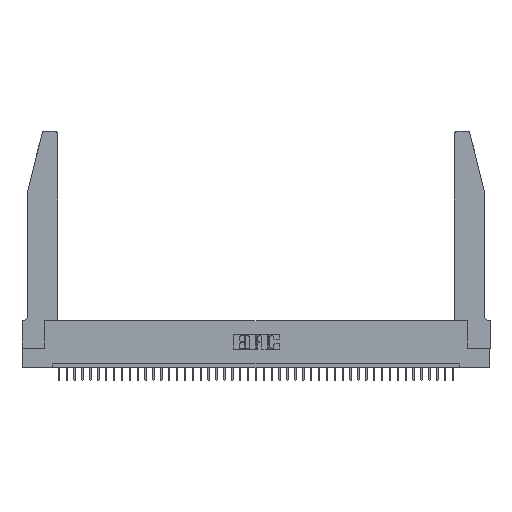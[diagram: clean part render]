
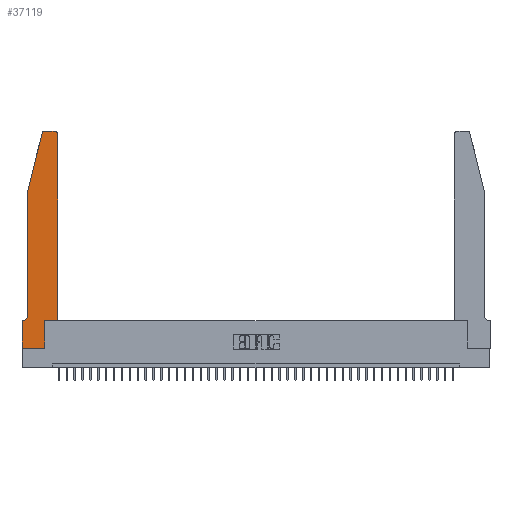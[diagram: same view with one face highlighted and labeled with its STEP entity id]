
A CAD part, top view. The second image highlights one B-rep face of the part: STEP entity #37119.
In plain terms, the highlighted planar face has unit normal (0, 0, 1).
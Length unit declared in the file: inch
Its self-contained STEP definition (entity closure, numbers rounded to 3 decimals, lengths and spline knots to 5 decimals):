
#324 = ORIENTED_EDGE ( 'NONE', *, *, #33193, .T. ) ;
#956 = CARTESIAN_POINT ( 'NONE',  ( 0.2865, 0.35, 0.37 ) ) ;
#963 = EDGE_CURVE ( 'NONE', #12908, #16970, #10690, .T. ) ;
#1066 = CARTESIAN_POINT ( 'NONE',  ( 0., 0., 0.37 ) ) ;
#1151 = CARTESIAN_POINT ( 'NONE',  ( 0., 0., 0.37 ) ) ;
#1848 = VECTOR ( 'NONE', #27713, 39.37008 ) ;
#1922 = DIRECTION ( 'NONE',  ( -1., 0., 0. ) ) ;
#2053 = VERTEX_POINT ( 'NONE', #23676 ) ;
#2090 = EDGE_CURVE ( 'NONE', #25463, #10935, #2439, .T. ) ;
#2155 = CARTESIAN_POINT ( 'NONE',  ( 0.2865, 0.35, 0.37 ) ) ;
#2161 = CARTESIAN_POINT ( 'NONE',  ( 0.0755, 2., 0.37 ) ) ;
#2421 = VERTEX_POINT ( 'NONE', #1151 ) ;
#2439 = CIRCLE ( 'NONE', #33643, 0.07 ) ;
#2647 = EDGE_CURVE ( 'NONE', #2421, #18058, #10616, .T. ) ;
#2859 = DIRECTION ( 'NONE',  ( 0., 0., 1. ) ) ;
#2985 = ORIENTED_EDGE ( 'NONE', *, *, #25477, .T. ) ;
#3070 = EDGE_CURVE ( 'NONE', #10935, #2053, #19215, .T. ) ;
#5065 = ORIENTED_EDGE ( 'NONE', *, *, #2647, .T. ) ;
#5070 = ORIENTED_EDGE ( 'NONE', *, *, #39161, .T. ) ;
#5489 = VECTOR ( 'NONE', #8986, 39.37008 ) ;
#5633 = VECTOR ( 'NONE', #26373, 39.37008 ) ;
#5861 = CARTESIAN_POINT ( 'NONE',  ( 0., 0., 0.37 ) ) ;
#6131 = VECTOR ( 'NONE', #7874, 39.37008 ) ;
#6667 = DIRECTION ( 'NONE',  ( 0., 0., 1. ) ) ;
#7221 = EDGE_LOOP ( 'NONE', ( #12255, #30014, #24522, #31162, #35668, #37573, #324, #5065, #5070, #12516, #27446, #2985 ) ) ;
#7874 = DIRECTION ( 'NONE',  ( 0., 1., 0. ) ) ;
#7950 = LINE ( 'NONE', #1066, #26227 ) ;
#8197 = CARTESIAN_POINT ( 'NONE',  ( 0.2865, 0., 0.37 ) ) ;
#8962 = VERTEX_POINT ( 'NONE', #33099 ) ;
#8986 = DIRECTION ( 'NONE',  ( -1., 0., 0. ) ) ;
#10113 = DIRECTION ( 'NONE',  ( 1., 0., 0. ) ) ;
#10242 = DIRECTION ( 'NONE',  ( 1., 0., 0. ) ) ;
#10523 = DIRECTION ( 'NONE',  ( 0., 0., 1. ) ) ;
#10616 = LINE ( 'NONE', #5861, #22814 ) ;
#10690 = LINE ( 'NONE', #33663, #6131 ) ;
#10935 = VERTEX_POINT ( 'NONE', #17726 ) ;
#11370 = CIRCLE ( 'NONE', #39183, 0.03 ) ;
#11614 = VERTEX_POINT ( 'NONE', #14839 ) ;
#12255 = ORIENTED_EDGE ( 'NONE', *, *, #16930, .T. ) ;
#12516 = ORIENTED_EDGE ( 'NONE', *, *, #23753, .T. ) ;
#12787 = DIRECTION ( 'NONE',  ( 1., 0., 0. ) ) ;
#12908 = VERTEX_POINT ( 'NONE', #32013 ) ;
#14839 = CARTESIAN_POINT ( 'NONE',  ( 0.25487, 2.72718, 0.37 ) ) ;
#14938 = CARTESIAN_POINT ( 'NONE',  ( 0.2605, 2.75, 0.37 ) ) ;
#15111 = CARTESIAN_POINT ( 'NONE',  ( 0.284, 2.75, 0.37 ) ) ;
#15152 = VERTEX_POINT ( 'NONE', #15111 ) ;
#15331 = DIRECTION ( 'NONE',  ( 0., -1., 0. ) ) ;
#15503 = CARTESIAN_POINT ( 'NONE',  ( 0.4505, 2.72, 0.37 ) ) ;
#16038 = CARTESIAN_POINT ( 'NONE',  ( 0.284, 2.72, 0.37 ) ) ;
#16930 = EDGE_CURVE ( 'NONE', #8962, #15152, #28844, .T. ) ;
#16970 = VERTEX_POINT ( 'NONE', #15503 ) ;
#17034 = PLANE ( 'NONE',  #22328 ) ;
#17726 = CARTESIAN_POINT ( 'NONE',  ( 0.0055, 0.35, 0.37 ) ) ;
#17908 = DIRECTION ( 'NONE',  ( 1., 0., 0. ) ) ;
#18058 = VERTEX_POINT ( 'NONE', #8197 ) ;
#19215 = LINE ( 'NONE', #30645, #26817 ) ;
#21968 = VECTOR ( 'NONE', #26940, 39.37008 ) ;
#22328 = AXIS2_PLACEMENT_3D ( 'NONE', #39568, #10523, #10242 ) ;
#22492 = CARTESIAN_POINT ( 'NONE',  ( 0.0755, 0.42, 0.37 ) ) ;
#22814 = VECTOR ( 'NONE', #17908, 39.37008 ) ;
#23544 = CARTESIAN_POINT ( 'NONE',  ( 0.0755, 2., 0.37 ) ) ;
#23676 = CARTESIAN_POINT ( 'NONE',  ( 0., 0.35, 0.37 ) ) ;
#23753 = EDGE_CURVE ( 'NONE', #27836, #12908, #27764, .T. ) ;
#23909 = LINE ( 'NONE', #23544, #5633 ) ;
#24251 = EDGE_CURVE ( 'NONE', #38512, #25463, #33740, .T. ) ;
#24522 = ORIENTED_EDGE ( 'NONE', *, *, #26906, .T. ) ;
#25158 = VECTOR ( 'NONE', #15331, 39.37008 ) ;
#25463 = VERTEX_POINT ( 'NONE', #22492 ) ;
#25477 = EDGE_CURVE ( 'NONE', #16970, #8962, #11370, .T. ) ;
#26227 = VECTOR ( 'NONE', #40353, 39.37008 ) ;
#26373 = DIRECTION ( 'NONE',  ( -0.239, -0.971, 0. ) ) ;
#26480 = CIRCLE ( 'NONE', #27012, 0.03 ) ;
#26491 = LINE ( 'NONE', #956, #21968 ) ;
#26817 = VECTOR ( 'NONE', #33894, 39.37008 ) ;
#26906 = EDGE_CURVE ( 'NONE', #11614, #38512, #23909, .T. ) ;
#26940 = DIRECTION ( 'NONE',  ( 0., 1., 0. ) ) ;
#27012 = AXIS2_PLACEMENT_3D ( 'NONE', #16038, #6667, #12787 ) ;
#27446 = ORIENTED_EDGE ( 'NONE', *, *, #963, .T. ) ;
#27713 = DIRECTION ( 'NONE',  ( 1., 0., 0. ) ) ;
#27727 = FACE_OUTER_BOUND ( 'NONE', #7221, .T. ) ;
#27764 = LINE ( 'NONE', #33781, #1848 ) ;
#27836 = VERTEX_POINT ( 'NONE', #2155 ) ;
#28844 = LINE ( 'NONE', #14938, #5489 ) ;
#30014 = ORIENTED_EDGE ( 'NONE', *, *, #41969, .T. ) ;
#30645 = CARTESIAN_POINT ( 'NONE',  ( 0.0755, 0.35, 0.37 ) ) ;
#31162 = ORIENTED_EDGE ( 'NONE', *, *, #24251, .T. ) ;
#31560 = CARTESIAN_POINT ( 'NONE',  ( 0.0055, 0.42, 0.37 ) ) ;
#32013 = CARTESIAN_POINT ( 'NONE',  ( 0.4505, 0.35, 0.37 ) ) ;
#33099 = CARTESIAN_POINT ( 'NONE',  ( 0.4205, 2.75, 0.37 ) ) ;
#33193 = EDGE_CURVE ( 'NONE', #2053, #2421, #7950, .T. ) ;
#33643 = AXIS2_PLACEMENT_3D ( 'NONE', #31560, #34250, #1922 ) ;
#33663 = CARTESIAN_POINT ( 'NONE',  ( 0.4505, 0.35, 0.37 ) ) ;
#33740 = LINE ( 'NONE', #37880, #25158 ) ;
#33781 = CARTESIAN_POINT ( 'NONE',  ( 0.4505, 0.35, 0.37 ) ) ;
#33894 = DIRECTION ( 'NONE',  ( -1., 0., 0. ) ) ;
#34250 = DIRECTION ( 'NONE',  ( 0., 0., -1. ) ) ;
#35668 = ORIENTED_EDGE ( 'NONE', *, *, #2090, .T. ) ;
#37119 = ADVANCED_FACE ( 'NONE', ( #27727 ), #17034, .T. ) ;
#37573 = ORIENTED_EDGE ( 'NONE', *, *, #3070, .T. ) ;
#37880 = CARTESIAN_POINT ( 'NONE',  ( 0.0755, 2., 0.37 ) ) ;
#38512 = VERTEX_POINT ( 'NONE', #2161 ) ;
#39161 = EDGE_CURVE ( 'NONE', #18058, #27836, #26491, .T. ) ;
#39183 = AXIS2_PLACEMENT_3D ( 'NONE', #41718, #2859, #10113 ) ;
#39568 = CARTESIAN_POINT ( 'NONE',  ( 0., 0.35, 0.37 ) ) ;
#40353 = DIRECTION ( 'NONE',  ( 0., -1., 0. ) ) ;
#41718 = CARTESIAN_POINT ( 'NONE',  ( 0.4205, 2.72, 0.37 ) ) ;
#41969 = EDGE_CURVE ( 'NONE', #15152, #11614, #26480, .T. ) ;
